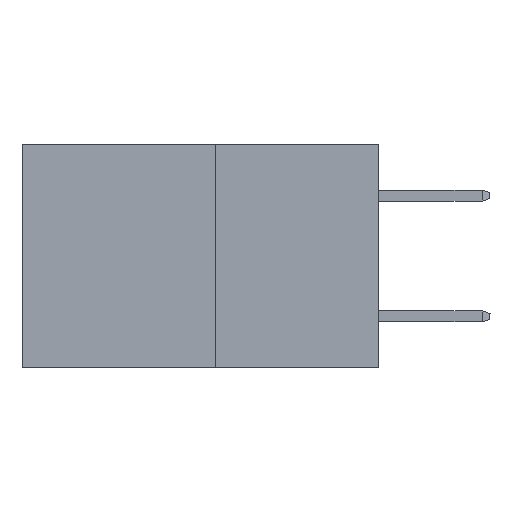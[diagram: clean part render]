
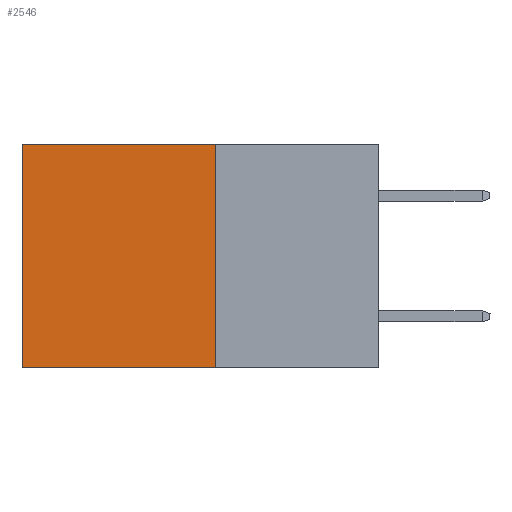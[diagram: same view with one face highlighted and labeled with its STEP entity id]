
A CAD part, left-side view. The second image highlights one B-rep face of the part: STEP entity #2546.
In plain terms, the highlighted planar face has unit normal (-1, 0, 0).
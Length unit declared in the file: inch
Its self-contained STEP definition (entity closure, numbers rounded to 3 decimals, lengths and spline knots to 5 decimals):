
#103 = EDGE_CURVE ( 'NONE', #8945, #5382, #9875, .T. ) ;
#261 = CARTESIAN_POINT ( 'NONE',  ( 0.277, 0.27, 0. ) ) ;
#682 = CARTESIAN_POINT ( 'NONE',  ( 0.277, 0.27, -0.37 ) ) ;
#748 = FACE_OUTER_BOUND ( 'NONE', #7424, .T. ) ;
#789 = ORIENTED_EDGE ( 'NONE', *, *, #8003, .F. ) ;
#886 = LINE ( 'NONE', #682, #7256 ) ;
#1075 = CARTESIAN_POINT ( 'NONE',  ( 0.277, 0.27, -0.37 ) ) ;
#1483 = CARTESIAN_POINT ( 'NONE',  ( 0.277, 0.59, 0. ) ) ;
#2332 = ORIENTED_EDGE ( 'NONE', *, *, #103, .F. ) ;
#2369 = DIRECTION ( 'NONE',  ( 0., 1., 0. ) ) ;
#2468 = CARTESIAN_POINT ( 'NONE',  ( 0.277, 0.59, -0.37 ) ) ;
#2519 = CARTESIAN_POINT ( 'NONE',  ( 0.277, 0.27, 0. ) ) ;
#2546 = ADVANCED_FACE ( 'NONE', ( #748 ), #3452, .F. ) ;
#3201 = DIRECTION ( 'NONE',  ( 1., 0., 0. ) ) ;
#3347 = LINE ( 'NONE', #2468, #5304 ) ;
#3394 = LINE ( 'NONE', #2519, #6151 ) ;
#3452 = PLANE ( 'NONE',  #9275 ) ;
#4026 = CARTESIAN_POINT ( 'NONE',  ( 0.277, 0.27, -0.37 ) ) ;
#4141 = DIRECTION ( 'NONE',  ( 0., 0., -1. ) ) ;
#4259 = EDGE_CURVE ( 'NONE', #8945, #6301, #3394, .T. ) ;
#4312 = CARTESIAN_POINT ( 'NONE',  ( 0.277, 0.27, -0.37 ) ) ;
#5304 = VECTOR ( 'NONE', #4141, 39.37008 ) ;
#5382 = VERTEX_POINT ( 'NONE', #1075 ) ;
#6143 = VECTOR ( 'NONE', #6682, 39.37008 ) ;
#6151 = VECTOR ( 'NONE', #9076, 39.37008 ) ;
#6301 = VERTEX_POINT ( 'NONE', #1483 ) ;
#6682 = DIRECTION ( 'NONE',  ( 0., 0., -1. ) ) ;
#7256 = VECTOR ( 'NONE', #2369, 39.37008 ) ;
#7424 = EDGE_LOOP ( 'NONE', ( #7929, #789, #2332, #10493 ) ) ;
#7929 = ORIENTED_EDGE ( 'NONE', *, *, #9973, .T. ) ;
#8003 = EDGE_CURVE ( 'NONE', #5382, #8787, #886, .T. ) ;
#8351 = CARTESIAN_POINT ( 'NONE',  ( 0.277, 0.59, -0.37 ) ) ;
#8787 = VERTEX_POINT ( 'NONE', #8351 ) ;
#8825 = DIRECTION ( 'NONE',  ( 0., 0., -1. ) ) ;
#8945 = VERTEX_POINT ( 'NONE', #261 ) ;
#9076 = DIRECTION ( 'NONE',  ( 0., 1., 0. ) ) ;
#9275 = AXIS2_PLACEMENT_3D ( 'NONE', #4026, #3201, #8825 ) ;
#9875 = LINE ( 'NONE', #4312, #6143 ) ;
#9973 = EDGE_CURVE ( 'NONE', #6301, #8787, #3347, .T. ) ;
#10493 = ORIENTED_EDGE ( 'NONE', *, *, #4259, .T. ) ;
